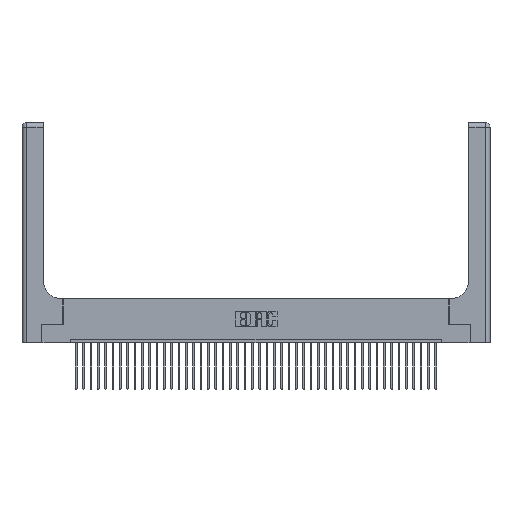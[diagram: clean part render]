
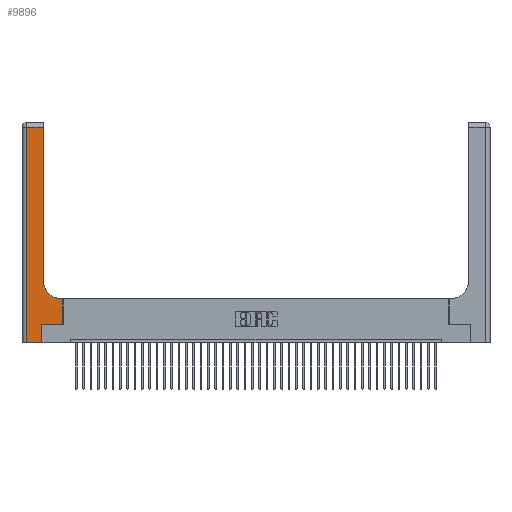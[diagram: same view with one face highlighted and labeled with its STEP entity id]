
A CAD part, top view. The second image highlights one B-rep face of the part: STEP entity #9896.
In plain terms, the highlighted planar face has unit normal (0, 0, 1).
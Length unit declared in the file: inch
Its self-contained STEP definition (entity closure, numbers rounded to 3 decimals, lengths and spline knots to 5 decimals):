
#455 = VERTEX_POINT ( 'NONE', #9938 ) ;
#459 = VERTEX_POINT ( 'NONE', #29625 ) ;
#1136 = DIRECTION ( 'NONE',  ( 0., 1., 0. ) ) ;
#1296 = CARTESIAN_POINT ( 'NONE',  ( 0.269, 0., 0.37 ) ) ;
#2079 = EDGE_CURVE ( 'NONE', #9153, #455, #22705, .T. ) ;
#2662 = EDGE_CURVE ( 'NONE', #5477, #9153, #19648, .T. ) ;
#2912 = PLANE ( 'NONE',  #14016 ) ;
#5173 = CARTESIAN_POINT ( 'NONE',  ( 0.06, 3., 0.37 ) ) ;
#5477 = VERTEX_POINT ( 'NONE', #12487 ) ;
#5738 = CARTESIAN_POINT ( 'NONE',  ( 0.5415, 0.85, 0.37 ) ) ;
#6032 = CARTESIAN_POINT ( 'NONE',  ( 0.269, 0.25, 0.37 ) ) ;
#7051 = VERTEX_POINT ( 'NONE', #17437 ) ;
#7616 = CARTESIAN_POINT ( 'NONE',  ( 0., 3., 0.37 ) ) ;
#7724 = EDGE_CURVE ( 'NONE', #455, #27386, #11437, .T. ) ;
#9109 = CARTESIAN_POINT ( 'NONE',  ( 0.2915, 0.85, 0.37 ) ) ;
#9153 = VERTEX_POINT ( 'NONE', #9109 ) ;
#9735 = VECTOR ( 'NONE', #1136, 39.37008 ) ;
#9896 = ADVANCED_FACE ( 'NONE', ( #13229 ), #2912, .F. ) ;
#9938 = CARTESIAN_POINT ( 'NONE',  ( 0.2915, 2.94, 0.37 ) ) ;
#11171 = VECTOR ( 'NONE', #24708, 39.37008 ) ;
#11437 = LINE ( 'NONE', #28749, #41678 ) ;
#12487 = CARTESIAN_POINT ( 'NONE',  ( 0.5415, 0.6, 0.37 ) ) ;
#13208 = LINE ( 'NONE', #5173, #41516 ) ;
#13229 = FACE_OUTER_BOUND ( 'NONE', #24178, .T. ) ;
#14005 = ORIENTED_EDGE ( 'NONE', *, *, #2662, .T. ) ;
#14016 = AXIS2_PLACEMENT_3D ( 'NONE', #7616, #38121, #15379 ) ;
#14463 = CARTESIAN_POINT ( 'NONE',  ( 0.06, 2.94, 0.37 ) ) ;
#14903 = DIRECTION ( 'NONE',  ( 1., 0., 0. ) ) ;
#15238 = ORIENTED_EDGE ( 'NONE', *, *, #22292, .T. ) ;
#15379 = DIRECTION ( 'NONE',  ( -1., 0., 0. ) ) ;
#15730 = VECTOR ( 'NONE', #28054, 39.37008 ) ;
#15973 = EDGE_CURVE ( 'NONE', #30695, #33417, #18326, .T. ) ;
#16203 = EDGE_CURVE ( 'NONE', #7051, #5477, #35413, .T. ) ;
#17437 = CARTESIAN_POINT ( 'NONE',  ( 0.5585, 0.6, 0.37 ) ) ;
#18277 = DIRECTION ( 'NONE',  ( 0., 0., -1. ) ) ;
#18326 = LINE ( 'NONE', #1296, #9735 ) ;
#18415 = DIRECTION ( 'NONE',  ( 0., -1., 0. ) ) ;
#19464 = VECTOR ( 'NONE', #26589, 39.37008 ) ;
#19648 = CIRCLE ( 'NONE', #39401, 0.25 ) ;
#19687 = EDGE_CURVE ( 'NONE', #27386, #459, #13208, .T. ) ;
#20076 = VECTOR ( 'NONE', #36759, 39.37008 ) ;
#20576 = VERTEX_POINT ( 'NONE', #38339 ) ;
#21887 = DIRECTION ( 'NONE',  ( -1., 0., 0. ) ) ;
#22167 = ORIENTED_EDGE ( 'NONE', *, *, #7724, .T. ) ;
#22292 = EDGE_CURVE ( 'NONE', #459, #30695, #37728, .T. ) ;
#22705 = LINE ( 'NONE', #34163, #11171 ) ;
#23287 = ORIENTED_EDGE ( 'NONE', *, *, #2079, .T. ) ;
#24178 = EDGE_LOOP ( 'NONE', ( #23287, #22167, #37865, #15238, #33669, #28949, #35358, #38519, #14005 ) ) ;
#24708 = DIRECTION ( 'NONE',  ( 0., 1., 0. ) ) ;
#26589 = DIRECTION ( 'NONE',  ( 1., 0., 0. ) ) ;
#27386 = VERTEX_POINT ( 'NONE', #14463 ) ;
#28054 = DIRECTION ( 'NONE',  ( 1., 0., 0. ) ) ;
#28699 = LINE ( 'NONE', #39701, #20076 ) ;
#28749 = CARTESIAN_POINT ( 'NONE',  ( 0., 2.94, 0.37 ) ) ;
#28949 = ORIENTED_EDGE ( 'NONE', *, *, #31601, .T. ) ;
#29625 = CARTESIAN_POINT ( 'NONE',  ( 0.06, 0., 0.37 ) ) ;
#30695 = VERTEX_POINT ( 'NONE', #36719 ) ;
#31601 = EDGE_CURVE ( 'NONE', #33417, #20576, #33324, .T. ) ;
#32384 = DIRECTION ( 'NONE',  ( -1., 0., 0. ) ) ;
#33123 = EDGE_CURVE ( 'NONE', #20576, #7051, #28699, .T. ) ;
#33324 = LINE ( 'NONE', #37406, #15730 ) ;
#33417 = VERTEX_POINT ( 'NONE', #6032 ) ;
#33669 = ORIENTED_EDGE ( 'NONE', *, *, #15973, .T. ) ;
#34163 = CARTESIAN_POINT ( 'NONE',  ( 0.2915, 3., 0.37 ) ) ;
#34966 = VECTOR ( 'NONE', #21887, 39.37008 ) ;
#35358 = ORIENTED_EDGE ( 'NONE', *, *, #33123, .T. ) ;
#35413 = LINE ( 'NONE', #38157, #34966 ) ;
#36719 = CARTESIAN_POINT ( 'NONE',  ( 0.269, 0., 0.37 ) ) ;
#36759 = DIRECTION ( 'NONE',  ( 0., 1., 0. ) ) ;
#37406 = CARTESIAN_POINT ( 'NONE',  ( 0.269, 0.25, 0.37 ) ) ;
#37728 = LINE ( 'NONE', #39596, #19464 ) ;
#37865 = ORIENTED_EDGE ( 'NONE', *, *, #19687, .T. ) ;
#38121 = DIRECTION ( 'NONE',  ( 0., 0., -1. ) ) ;
#38157 = CARTESIAN_POINT ( 'NONE',  ( 0.2915, 0.6, 0.37 ) ) ;
#38339 = CARTESIAN_POINT ( 'NONE',  ( 0.5585, 0.25, 0.37 ) ) ;
#38519 = ORIENTED_EDGE ( 'NONE', *, *, #16203, .T. ) ;
#39401 = AXIS2_PLACEMENT_3D ( 'NONE', #5738, #18277, #14903 ) ;
#39596 = CARTESIAN_POINT ( 'NONE',  ( 0., 0., 0.37 ) ) ;
#39701 = CARTESIAN_POINT ( 'NONE',  ( 0.5585, 0.25, 0.37 ) ) ;
#41516 = VECTOR ( 'NONE', #18415, 39.37008 ) ;
#41678 = VECTOR ( 'NONE', #32384, 39.37008 ) ;
